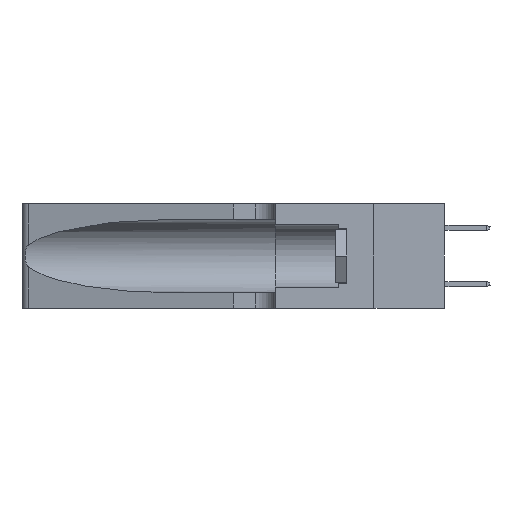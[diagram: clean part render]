
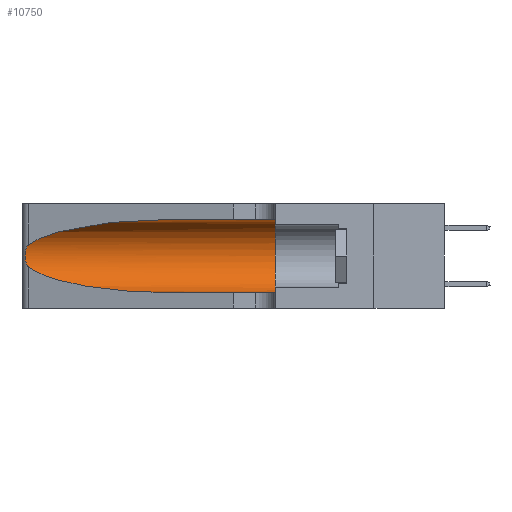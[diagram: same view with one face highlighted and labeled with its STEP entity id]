
A CAD part, left-side view. The second image highlights one B-rep face of the part: STEP entity #10750.
In plain terms, the highlighted cylindrical face has radius 3.308 mm (diameter 6.617 mm), a partial arc.
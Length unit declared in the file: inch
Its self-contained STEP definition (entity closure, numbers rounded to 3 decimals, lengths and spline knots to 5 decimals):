
#263 = CARTESIAN_POINT ( 'NONE',  ( 0.25487, 1.22718, 0.14631 ) ) ;
#889 = CARTESIAN_POINT ( 'NONE',  ( 0.1305, 1.61858, 0.31525 ) ) ;
#930 = VERTEX_POINT ( 'NONE', #17978 ) ;
#1071 = EDGE_LOOP ( 'NONE', ( #15227, #13294, #7938, #12127, #33289, #34950 ) ) ;
#1735 = CARTESIAN_POINT ( 'NONE',  ( 0.18966, 0.96281, 0.31525 ) ) ;
#2931 = CARTESIAN_POINT ( 'NONE',  ( 0.25639, 1.23184, 0.21858 ) ) ;
#4073 = CARTESIAN_POINT ( 'NONE',  ( 0.1305, 1.61858, 0.05475 ) ) ;
#4400 = LINE ( 'NONE', #889, #32407 ) ;
#4448 = AXIS2_PLACEMENT_3D ( 'NONE', #7911, #34924, #5152 ) ;
#4477 = CARTESIAN_POINT ( 'NONE',  ( 0.2373, 1.15595, 0.28018 ) ) ;
#5152 = DIRECTION ( 'NONE',  ( 0., 0., -1. ) ) ;
#5674 = CARTESIAN_POINT ( 'NONE',  ( 0.25854, 1.2359, 0.20912 ) ) ;
#6412 =( BOUNDED_CURVE ( )  B_SPLINE_CURVE ( 3, ( #34254, #1735, #4477, #23515 ),
 .UNSPECIFIED., .F., .T. ) 
 B_SPLINE_CURVE_WITH_KNOTS ( ( 4, 4 ),
 ( 1.5708, 2.84003 ),
 .UNSPECIFIED. ) 
 CURVE ( )  GEOMETRIC_REPRESENTATION_ITEM ( )  RATIONAL_B_SPLINE_CURVE ( ( 1., 0.87, 0.87, 1. ) ) 
 REPRESENTATION_ITEM ( '' )  );
#6506 = DIRECTION ( 'NONE',  ( 0., -1., 0. ) ) ;
#6810 = EDGE_CURVE ( 'NONE', #23012, #34897, #28506, .T. ) ;
#6812 = VERTEX_POINT ( 'NONE', #9561 ) ;
#6817 = DIRECTION ( 'NONE',  ( 0., -1., 0. ) ) ;
#6918 = CARTESIAN_POINT ( 'NONE',  ( 0.1305, 0.72297, 0.05475 ) ) ;
#7911 = CARTESIAN_POINT ( 'NONE',  ( 0.1305, 1.61858, 0.185 ) ) ;
#7922 = EDGE_CURVE ( 'NONE', #930, #6812, #15400, .T. ) ;
#7938 = ORIENTED_EDGE ( 'NONE', *, *, #13384, .T. ) ;
#8422 = CARTESIAN_POINT ( 'NONE',  ( 0.26075, 1.23896, 0.19203 ) ) ;
#9245 = VERTEX_POINT ( 'NONE', #24984 ) ;
#9561 = CARTESIAN_POINT ( 'NONE',  ( 0.25487, 1.22718, 0.14631 ) ) ;
#10242 = CARTESIAN_POINT ( 'NONE',  ( 0.1305, 0.35, 0.05475 ) ) ;
#10750 = ADVANCED_FACE ( 'NONE', ( #21952 ), #28288, .F. ) ;
#11170 = CARTESIAN_POINT ( 'NONE',  ( 0.26017, 1.23833, 0.17102 ) ) ;
#12127 = ORIENTED_EDGE ( 'NONE', *, *, #6810, .T. ) ;
#12691 = DIRECTION ( 'NONE',  ( 0., 1., 0. ) ) ;
#13294 = ORIENTED_EDGE ( 'NONE', *, *, #7922, .T. ) ;
#13384 = EDGE_CURVE ( 'NONE', #6812, #23012, #31652, .T. ) ;
#13677 = CARTESIAN_POINT ( 'NONE',  ( 0.25555, 1.22994, 0.2215 ) ) ;
#13921 = CARTESIAN_POINT ( 'NONE',  ( 0.25789, 1.23486, 0.15765 ) ) ;
#15037 = CARTESIAN_POINT ( 'NONE',  ( 0.2373, 1.15595, 0.08982 ) ) ;
#15227 = ORIENTED_EDGE ( 'NONE', *, *, #28330, .T. ) ;
#15400 = B_SPLINE_CURVE_WITH_KNOTS ( 'NONE', 3,
 ( #29913, #13677, #2931, #21984, #5674, #24707, #8422, #27399, #11170, #30142, #13921, #32829, #16658, #263 ),
 .UNSPECIFIED., .F., .F.,
 ( 4, 2, 2, 2, 2, 2, 4 ),
 ( 0., 0.00027, 0.00053, 0.00107, 0.0016, 0.00187, 0.00214 ),
 .UNSPECIFIED. ) ;
#16658 = CARTESIAN_POINT ( 'NONE',  ( 0.25555, 1.22993, 0.14849 ) ) ;
#17057 = CARTESIAN_POINT ( 'NONE',  ( 0.1305, 0.72297, 0.05475 ) ) ;
#17978 = CARTESIAN_POINT ( 'NONE',  ( 0.25487, 1.22718, 0.22369 ) ) ;
#18521 = EDGE_CURVE ( 'NONE', #33138, #9245, #4400, .T. ) ;
#21952 = FACE_OUTER_BOUND ( 'NONE', #1071, .T. ) ;
#21984 = CARTESIAN_POINT ( 'NONE',  ( 0.25787, 1.23484, 0.2124 ) ) ;
#23012 = VERTEX_POINT ( 'NONE', #17057 ) ;
#23223 = CARTESIAN_POINT ( 'NONE',  ( 0.18966, 0.96281, 0.05475 ) ) ;
#23515 = CARTESIAN_POINT ( 'NONE',  ( 0.25487, 1.22718, 0.22369 ) ) ;
#24707 = CARTESIAN_POINT ( 'NONE',  ( 0.26018, 1.23835, 0.19895 ) ) ;
#24984 = CARTESIAN_POINT ( 'NONE',  ( 0.1305, 0.35, 0.31525 ) ) ;
#27344 = CARTESIAN_POINT ( 'NONE',  ( 0.1305, 0.72297, 0.31525 ) ) ;
#27399 = CARTESIAN_POINT ( 'NONE',  ( 0.26075, 1.23896, 0.178 ) ) ;
#27650 = VECTOR ( 'NONE', #6817, 39.37008 ) ;
#28288 = CYLINDRICAL_SURFACE ( 'NONE', #4448, 0.13025 ) ;
#28330 = EDGE_CURVE ( 'NONE', #33138, #930, #6412, .T. ) ;
#28506 = LINE ( 'NONE', #4073, #27650 ) ;
#28777 = CIRCLE ( 'NONE', #31375, 0.13025 ) ;
#28908 = CARTESIAN_POINT ( 'NONE',  ( 0.1305, 0.35, 0.185 ) ) ;
#29913 = CARTESIAN_POINT ( 'NONE',  ( 0.25487, 1.22718, 0.22369 ) ) ;
#30142 = CARTESIAN_POINT ( 'NONE',  ( 0.25856, 1.23593, 0.16098 ) ) ;
#31375 = AXIS2_PLACEMENT_3D ( 'NONE', #28908, #12691, #31617 ) ;
#31617 = DIRECTION ( 'NONE',  ( 0., 0., 1. ) ) ;
#31652 =( BOUNDED_CURVE ( )  B_SPLINE_CURVE ( 3, ( #33948, #15037, #23223, #6918 ),
 .UNSPECIFIED., .F., .T. ) 
 B_SPLINE_CURVE_WITH_KNOTS ( ( 4, 4 ),
 ( 3.44316, 4.71239 ),
 .UNSPECIFIED. ) 
 CURVE ( )  GEOMETRIC_REPRESENTATION_ITEM ( )  RATIONAL_B_SPLINE_CURVE ( ( 1., 0.87, 0.87, 1. ) ) 
 REPRESENTATION_ITEM ( '' )  );
#32407 = VECTOR ( 'NONE', #6506, 39.37008 ) ;
#32829 = CARTESIAN_POINT ( 'NONE',  ( 0.25639, 1.23186, 0.15144 ) ) ;
#32875 = EDGE_CURVE ( 'NONE', #9245, #34897, #28777, .T. ) ;
#33138 = VERTEX_POINT ( 'NONE', #27344 ) ;
#33289 = ORIENTED_EDGE ( 'NONE', *, *, #32875, .F. ) ;
#33948 = CARTESIAN_POINT ( 'NONE',  ( 0.25487, 1.22718, 0.14631 ) ) ;
#34254 = CARTESIAN_POINT ( 'NONE',  ( 0.1305, 0.72297, 0.31525 ) ) ;
#34897 = VERTEX_POINT ( 'NONE', #10242 ) ;
#34924 = DIRECTION ( 'NONE',  ( 0., -1., 0. ) ) ;
#34950 = ORIENTED_EDGE ( 'NONE', *, *, #18521, .F. ) ;
